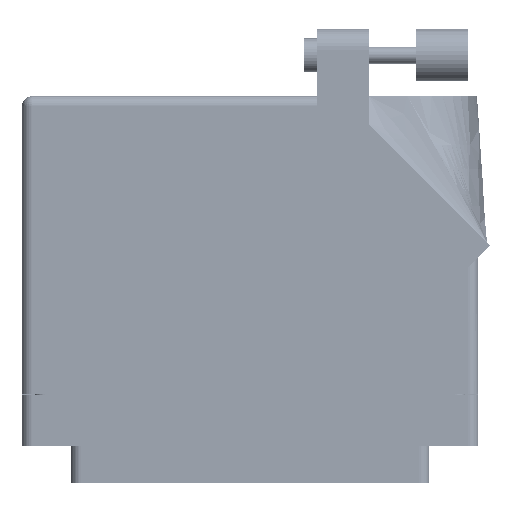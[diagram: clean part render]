
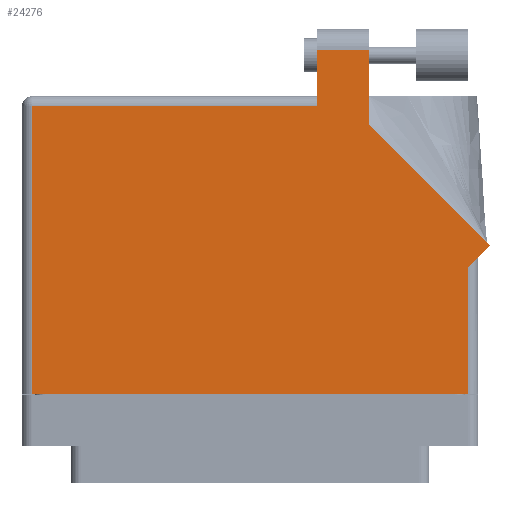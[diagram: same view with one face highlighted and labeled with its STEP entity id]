
A CAD part, front view. The second image highlights one B-rep face of the part: STEP entity #24276.
In plain terms, the highlighted face is planar.
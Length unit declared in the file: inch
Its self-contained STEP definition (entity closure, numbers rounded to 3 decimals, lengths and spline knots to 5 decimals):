
#62 = VECTOR ( 'NONE', #42033, 39.37008 ) ;
#1180 = VERTEX_POINT ( 'NONE', #15623 ) ;
#2061 = ORIENTED_EDGE ( 'NONE', *, *, #52032, .T. ) ;
#3727 = CARTESIAN_POINT ( 'NONE',  ( 1.42971, 0.78571, 0.617 ) ) ;
#4040 = CARTESIAN_POINT ( 'NONE',  ( 1.297, 0.715, 0.617 ) ) ;
#4868 = EDGE_CURVE ( 'NONE', #1180, #54342, #19680, .T. ) ;
#5134 = EDGE_CURVE ( 'NONE', #67424, #41207, #45912, .T. ) ;
#5399 = LINE ( 'NONE', #5755, #34858 ) ;
#5755 = CARTESIAN_POINT ( 'NONE',  ( 1.42971, 0.78571, 0.617 ) ) ;
#7693 = VECTOR ( 'NONE', #45849, 39.37008 ) ;
#9379 = ORIENTED_EDGE ( 'NONE', *, *, #37252, .T. ) ;
#9389 = LINE ( 'NONE', #4040, #32494 ) ;
#10213 = CARTESIAN_POINT ( 'NONE',  ( -1.297, 1.613, 0.617 ) ) ;
#10651 = LINE ( 'NONE', #32380, #7693 ) ;
#10703 = ORIENTED_EDGE ( 'NONE', *, *, #52162, .T. ) ;
#11038 = DIRECTION ( 'NONE',  ( 0., 1., 0. ) ) ;
#12879 = DIRECTION ( 'NONE',  ( -1., 0., 0. ) ) ;
#13191 = VECTOR ( 'NONE', #35569, 39.37008 ) ;
#13263 = CARTESIAN_POINT ( 'NONE',  ( -1.359, -0.1, 0.617 ) ) ;
#13339 = CARTESIAN_POINT ( 'NONE',  ( 0.706, 1.95, 0.617 ) ) ;
#14338 = CARTESIAN_POINT ( 'NONE',  ( 1.359, 0.715, 0.617 ) ) ;
#14429 = LINE ( 'NONE', #25098, #22784 ) ;
#15623 = CARTESIAN_POINT ( 'NONE',  ( 1.297, 0.653, 0.617 ) ) ;
#18220 = DIRECTION ( 'NONE',  ( 0., 0., -1. ) ) ;
#18936 = LINE ( 'NONE', #61243, #55576 ) ;
#19680 = LINE ( 'NONE', #14338, #26297 ) ;
#20811 = EDGE_CURVE ( 'NONE', #53074, #67424, #18936, .T. ) ;
#21069 = DIRECTION ( 'NONE',  ( -0.707, 0.707, 0. ) ) ;
#22784 = VECTOR ( 'NONE', #46778, 39.37008 ) ;
#24276 = ADVANCED_FACE ( 'NONE', ( #60207 ), #34592, .F. ) ;
#24571 = CARTESIAN_POINT ( 'NONE',  ( 0.399, 1.675, 0.617 ) ) ;
#24878 = CARTESIAN_POINT ( 'NONE',  ( -1.297, -0.1, 0.617 ) ) ;
#24907 = ORIENTED_EDGE ( 'NONE', *, *, #4868, .T. ) ;
#25098 = CARTESIAN_POINT ( 'NONE',  ( -1.359, 1.613, 0.617 ) ) ;
#25887 = VERTEX_POINT ( 'NONE', #10213 ) ;
#26297 = VECTOR ( 'NONE', #36039, 39.37008 ) ;
#28732 = VERTEX_POINT ( 'NONE', #53891 ) ;
#29437 = AXIS2_PLACEMENT_3D ( 'NONE', #39919, #18220, #61593 ) ;
#32380 = CARTESIAN_POINT ( 'NONE',  ( 0.706, 1.50942, 0.617 ) ) ;
#32494 = VECTOR ( 'NONE', #11038, 39.37008 ) ;
#34592 = PLANE ( 'NONE',  #29437 ) ;
#34858 = VECTOR ( 'NONE', #21069, 39.37008 ) ;
#35029 = EDGE_CURVE ( 'NONE', #52722, #53074, #10651, .T. ) ;
#35569 = DIRECTION ( 'NONE',  ( 0., -1., 0. ) ) ;
#36039 = DIRECTION ( 'NONE',  ( 0.707, 0.707, 0. ) ) ;
#36260 = LINE ( 'NONE', #24878, #13191 ) ;
#37252 = EDGE_CURVE ( 'NONE', #54342, #52722, #5399, .T. ) ;
#39919 = CARTESIAN_POINT ( 'NONE',  ( -1.359, 1.675, 0.617 ) ) ;
#41207 = VERTEX_POINT ( 'NONE', #48815 ) ;
#41497 = CARTESIAN_POINT ( 'NONE',  ( 0.706, 1.50942, 0.617 ) ) ;
#42033 = DIRECTION ( 'NONE',  ( 1., 0., 0. ) ) ;
#42549 = ORIENTED_EDGE ( 'NONE', *, *, #58603, .T. ) ;
#43232 = ORIENTED_EDGE ( 'NONE', *, *, #5134, .T. ) ;
#43919 = EDGE_CURVE ( 'NONE', #66501, #28732, #61974, .T. ) ;
#44723 = EDGE_LOOP ( 'NONE', ( #58313, #63981, #43232, #42549, #10703, #60325, #2061, #24907, #9379 ) ) ;
#45849 = DIRECTION ( 'NONE',  ( 0., 1., 0. ) ) ;
#45912 = LINE ( 'NONE', #24571, #62505 ) ;
#46261 = DIRECTION ( 'NONE',  ( 0., -1., 0. ) ) ;
#46778 = DIRECTION ( 'NONE',  ( -1., 0., 0. ) ) ;
#48815 = CARTESIAN_POINT ( 'NONE',  ( 0.399, 1.613, 0.617 ) ) ;
#49094 = CARTESIAN_POINT ( 'NONE',  ( 0.399, 1.95, 0.617 ) ) ;
#52032 = EDGE_CURVE ( 'NONE', #28732, #1180, #9389, .T. ) ;
#52162 = EDGE_CURVE ( 'NONE', #25887, #66501, #36260, .T. ) ;
#52722 = VERTEX_POINT ( 'NONE', #41497 ) ;
#53074 = VERTEX_POINT ( 'NONE', #13339 ) ;
#53891 = CARTESIAN_POINT ( 'NONE',  ( 1.297, -0.1, 0.617 ) ) ;
#54342 = VERTEX_POINT ( 'NONE', #3727 ) ;
#55576 = VECTOR ( 'NONE', #12879, 39.37008 ) ;
#57233 = CARTESIAN_POINT ( 'NONE',  ( -1.297, -0.1, 0.617 ) ) ;
#58313 = ORIENTED_EDGE ( 'NONE', *, *, #35029, .T. ) ;
#58603 = EDGE_CURVE ( 'NONE', #41207, #25887, #14429, .T. ) ;
#60207 = FACE_OUTER_BOUND ( 'NONE', #44723, .T. ) ;
#60325 = ORIENTED_EDGE ( 'NONE', *, *, #43919, .T. ) ;
#61243 = CARTESIAN_POINT ( 'NONE',  ( 0.399, 1.95, 0.617 ) ) ;
#61593 = DIRECTION ( 'NONE',  ( -1., 0., 0. ) ) ;
#61974 = LINE ( 'NONE', #13263, #62 ) ;
#62505 = VECTOR ( 'NONE', #46261, 39.37008 ) ;
#63981 = ORIENTED_EDGE ( 'NONE', *, *, #20811, .T. ) ;
#66501 = VERTEX_POINT ( 'NONE', #57233 ) ;
#67424 = VERTEX_POINT ( 'NONE', #49094 ) ;
